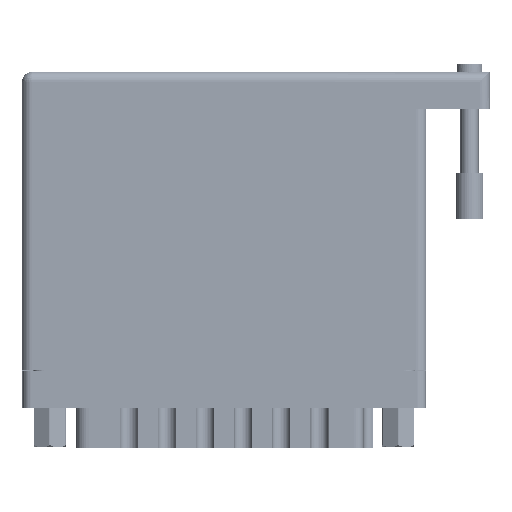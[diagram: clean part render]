
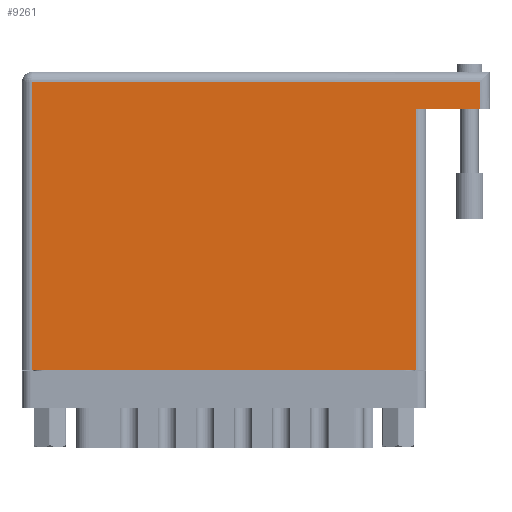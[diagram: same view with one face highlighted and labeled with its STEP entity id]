
A CAD part, front view. The second image highlights one B-rep face of the part: STEP entity #9261.
In plain terms, the highlighted face is planar.
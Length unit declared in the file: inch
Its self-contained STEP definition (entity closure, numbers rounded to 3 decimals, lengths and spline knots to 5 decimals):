
#2475 = LINE ( 'NONE', #3938, #20530 ) ;
#3938 = CARTESIAN_POINT ( 'NONE',  ( 3.12, 2.03, 0. ) ) ;
#6669 = EDGE_CURVE ( 'NONE', #11854, #22958, #2475, .T. ) ;
#8316 = DIRECTION ( 'NONE',  ( -1., 0., 0. ) ) ;
#8421 = CARTESIAN_POINT ( 'NONE',  ( 0.07, 1.96, 0. ) ) ;
#9261 = ADVANCED_FACE ( 'NONE', ( #48173 ), #39762, .F. ) ;
#9610 = VERTEX_POINT ( 'NONE', #8421 ) ;
#9715 = VERTEX_POINT ( 'NONE', #60199 ) ;
#11854 = VERTEX_POINT ( 'NONE', #72939 ) ;
#14747 = VECTOR ( 'NONE', #48098, 39.37008 ) ;
#15564 = CARTESIAN_POINT ( 'NONE',  ( 0.07, 0., 0. ) ) ;
#16336 = ORIENTED_EDGE ( 'NONE', *, *, #73066, .F. ) ;
#17264 = CARTESIAN_POINT ( 'NONE',  ( 0., 1.96, 0. ) ) ;
#20530 = VECTOR ( 'NONE', #61162, 39.37008 ) ;
#22958 = VERTEX_POINT ( 'NONE', #101775 ) ;
#23878 = LINE ( 'NONE', #17264, #57026 ) ;
#24235 = ORIENTED_EDGE ( 'NONE', *, *, #6669, .T. ) ;
#26332 = AXIS2_PLACEMENT_3D ( 'NONE', #65110, #105601, #8316 ) ;
#30889 = CARTESIAN_POINT ( 'NONE',  ( 2.685, 0., 0. ) ) ;
#38574 = EDGE_CURVE ( 'NONE', #66898, #71684, #50303, .T. ) ;
#39762 = PLANE ( 'NONE',  #26332 ) ;
#41119 = EDGE_CURVE ( 'NONE', #71684, #9715, #99805, .T. ) ;
#45109 = CARTESIAN_POINT ( 'NONE',  ( 0.07, 0., 0. ) ) ;
#46113 = VECTOR ( 'NONE', #58962, 39.37008 ) ;
#46951 = ORIENTED_EDGE ( 'NONE', *, *, #105946, .T. ) ;
#47324 = EDGE_LOOP ( 'NONE', ( #48017, #102775, #16336, #24235, #93988, #46951 ) ) ;
#48017 = ORIENTED_EDGE ( 'NONE', *, *, #38574, .T. ) ;
#48098 = DIRECTION ( 'NONE',  ( -1., 0., 0. ) ) ;
#48173 = FACE_OUTER_BOUND ( 'NONE', #47324, .T. ) ;
#50303 = LINE ( 'NONE', #100094, #78464 ) ;
#55543 = DIRECTION ( 'NONE',  ( 0., -1., 0. ) ) ;
#57026 = VECTOR ( 'NONE', #75824, 39.37008 ) ;
#57190 = VECTOR ( 'NONE', #55543, 39.37008 ) ;
#58962 = DIRECTION ( 'NONE',  ( 0., 1., 0. ) ) ;
#60199 = CARTESIAN_POINT ( 'NONE',  ( 2.685, 1.774, 0. ) ) ;
#61162 = DIRECTION ( 'NONE',  ( 0., 1., 0. ) ) ;
#65110 = CARTESIAN_POINT ( 'NONE',  ( 0., 2.03, 0. ) ) ;
#66898 = VERTEX_POINT ( 'NONE', #45109 ) ;
#69958 = LINE ( 'NONE', #15564, #57190 ) ;
#71684 = VERTEX_POINT ( 'NONE', #30889 ) ;
#72939 = CARTESIAN_POINT ( 'NONE',  ( 3.12, 1.774, 0. ) ) ;
#73066 = EDGE_CURVE ( 'NONE', #11854, #9715, #90200, .T. ) ;
#75429 = DIRECTION ( 'NONE',  ( 1., 0., 0. ) ) ;
#75800 = CARTESIAN_POINT ( 'NONE',  ( 2.685, 1.774, 0. ) ) ;
#75824 = DIRECTION ( 'NONE',  ( -1., 0., 0. ) ) ;
#78464 = VECTOR ( 'NONE', #75429, 39.37008 ) ;
#86062 = EDGE_CURVE ( 'NONE', #22958, #9610, #23878, .T. ) ;
#90200 = LINE ( 'NONE', #98179, #14747 ) ;
#93988 = ORIENTED_EDGE ( 'NONE', *, *, #86062, .T. ) ;
#98179 = CARTESIAN_POINT ( 'NONE',  ( 3.19, 1.774, 0. ) ) ;
#99805 = LINE ( 'NONE', #75800, #46113 ) ;
#100094 = CARTESIAN_POINT ( 'NONE',  ( 0., 0., 0. ) ) ;
#101775 = CARTESIAN_POINT ( 'NONE',  ( 3.12, 1.96, 0. ) ) ;
#102775 = ORIENTED_EDGE ( 'NONE', *, *, #41119, .T. ) ;
#105601 = DIRECTION ( 'NONE',  ( 0., 0., -1. ) ) ;
#105946 = EDGE_CURVE ( 'NONE', #9610, #66898, #69958, .T. ) ;
